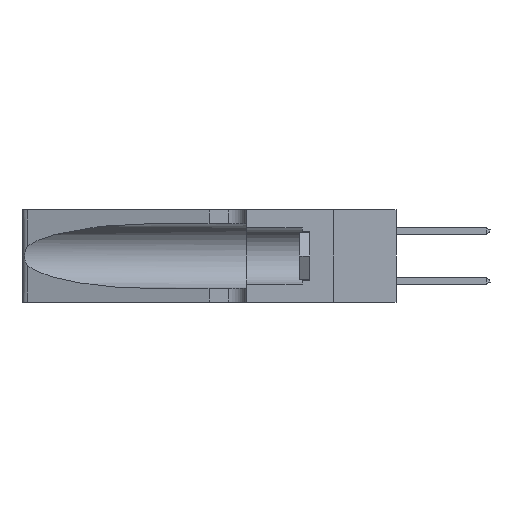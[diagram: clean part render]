
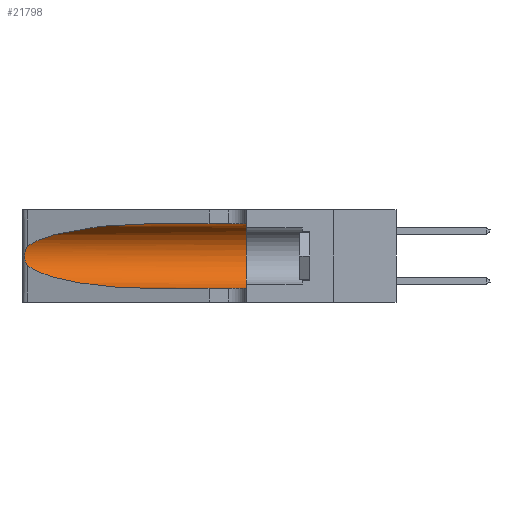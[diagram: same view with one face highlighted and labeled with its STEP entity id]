
A CAD part, left-side view. The second image highlights one B-rep face of the part: STEP entity #21798.
In plain terms, the highlighted cylindrical face has radius 3.308 mm (diameter 6.617 mm), a partial arc.
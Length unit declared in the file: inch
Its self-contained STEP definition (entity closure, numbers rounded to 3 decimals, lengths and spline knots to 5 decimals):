
#53 = CARTESIAN_POINT ( 'NONE',  ( 0.1305, 1.61858, 0.05475 ) ) ;
#1114 = CARTESIAN_POINT ( 'NONE',  ( 0.26075, 1.23896, 0.19203 ) ) ;
#1781 =( BOUNDED_CURVE ( )  B_SPLINE_CURVE ( 3, ( #29916, #9911, #32738, #15799 ),
 .UNSPECIFIED., .F., .F. ) 
 B_SPLINE_CURVE_WITH_KNOTS ( ( 4, 4 ),
 ( 1.5708, 2.84003 ),
 .UNSPECIFIED. ) 
 CURVE ( )  GEOMETRIC_REPRESENTATION_ITEM ( )  RATIONAL_B_SPLINE_CURVE ( ( 1., 0.87, 0.87, 1. ) ) 
 REPRESENTATION_ITEM ( '' )  );
#2050 = AXIS2_PLACEMENT_3D ( 'NONE', #6379, #26395, #9287 ) ;
#2998 = EDGE_LOOP ( 'NONE', ( #20189, #3966, #34275, #18546, #19364, #13245 ) ) ;
#3966 = ORIENTED_EDGE ( 'NONE', *, *, #14239, .T. ) ;
#4120 = CARTESIAN_POINT ( 'NONE',  ( 0.26017, 1.23833, 0.17102 ) ) ;
#4672 = B_SPLINE_CURVE_WITH_KNOTS ( 'NONE', 3,
 ( #24072, #9840, #32544, #15597, #35403, #18487, #1114, #21344, #4120, #24201, #7073, #27046, #9971, #29843 ),
 .UNSPECIFIED., .F., .F.,
 ( 4, 2, 2, 2, 2, 2, 4 ),
 ( 0., 0.00027, 0.00053, 0.00107, 0.0016, 0.00187, 0.00214 ),
 .UNSPECIFIED. ) ;
#4961 = VERTEX_POINT ( 'NONE', #33098 ) ;
#5227 = VERTEX_POINT ( 'NONE', #11500 ) ;
#5670 = CARTESIAN_POINT ( 'NONE',  ( 0.1305, 1.61858, 0.31525 ) ) ;
#6115 = CARTESIAN_POINT ( 'NONE',  ( 0.1305, 0.72297, 0.05475 ) ) ;
#6379 = CARTESIAN_POINT ( 'NONE',  ( 0.1305, 0.35, 0.185 ) ) ;
#7073 = CARTESIAN_POINT ( 'NONE',  ( 0.25789, 1.23486, 0.15765 ) ) ;
#9287 = DIRECTION ( 'NONE',  ( 0., 0., 1. ) ) ;
#9401 = CARTESIAN_POINT ( 'NONE',  ( 0.1305, 1.61858, 0.185 ) ) ;
#9840 = CARTESIAN_POINT ( 'NONE',  ( 0.25555, 1.22994, 0.2215 ) ) ;
#9911 = CARTESIAN_POINT ( 'NONE',  ( 0.18966, 0.96281, 0.31525 ) ) ;
#9971 = CARTESIAN_POINT ( 'NONE',  ( 0.25555, 1.22993, 0.14849 ) ) ;
#10057 = EDGE_CURVE ( 'NONE', #14103, #4961, #18023, .T. ) ;
#11257 = CARTESIAN_POINT ( 'NONE',  ( 0.1305, 0.35, 0.31525 ) ) ;
#11417 = CARTESIAN_POINT ( 'NONE',  ( 0.25487, 1.22718, 0.22369 ) ) ;
#11500 = CARTESIAN_POINT ( 'NONE',  ( 0.1305, 0.72297, 0.31525 ) ) ;
#11599 = CARTESIAN_POINT ( 'NONE',  ( 0.25487, 1.22718, 0.14631 ) ) ;
#12283 = DIRECTION ( 'NONE',  ( 0., -1., 0. ) ) ;
#13133 = CYLINDRICAL_SURFACE ( 'NONE', #27739, 0.13025 ) ;
#13245 = ORIENTED_EDGE ( 'NONE', *, *, #31422, .F. ) ;
#14103 = VERTEX_POINT ( 'NONE', #11599 ) ;
#14217 = DIRECTION ( 'NONE',  ( 0., -1., 0. ) ) ;
#14239 = EDGE_CURVE ( 'NONE', #15331, #14103, #4672, .T. ) ;
#14615 = DIRECTION ( 'NONE',  ( 0., -1., 0. ) ) ;
#14776 = VERTEX_POINT ( 'NONE', #23659 ) ;
#15331 = VERTEX_POINT ( 'NONE', #11417 ) ;
#15597 = CARTESIAN_POINT ( 'NONE',  ( 0.25787, 1.23484, 0.2124 ) ) ;
#15799 = CARTESIAN_POINT ( 'NONE',  ( 0.25487, 1.22718, 0.22369 ) ) ;
#18023 =( BOUNDED_CURVE ( )  B_SPLINE_CURVE ( 3, ( #26009, #23145, #23266, #6115 ),
 .UNSPECIFIED., .F., .T. ) 
 B_SPLINE_CURVE_WITH_KNOTS ( ( 4, 4 ),
 ( 3.44316, 4.71239 ),
 .UNSPECIFIED. ) 
 CURVE ( )  GEOMETRIC_REPRESENTATION_ITEM ( )  RATIONAL_B_SPLINE_CURVE ( ( 1., 0.87, 0.87, 1. ) ) 
 REPRESENTATION_ITEM ( '' )  );
#18487 = CARTESIAN_POINT ( 'NONE',  ( 0.26018, 1.23835, 0.19895 ) ) ;
#18546 = ORIENTED_EDGE ( 'NONE', *, *, #20034, .T. ) ;
#19364 = ORIENTED_EDGE ( 'NONE', *, *, #35878, .F. ) ;
#19437 = CIRCLE ( 'NONE', #2050, 0.13025 ) ;
#20034 = EDGE_CURVE ( 'NONE', #4961, #14776, #27897, .T. ) ;
#20189 = ORIENTED_EDGE ( 'NONE', *, *, #25973, .T. ) ;
#21055 = LINE ( 'NONE', #5670, #27699 ) ;
#21344 = CARTESIAN_POINT ( 'NONE',  ( 0.26075, 1.23896, 0.178 ) ) ;
#21798 = ADVANCED_FACE ( 'NONE', ( #35739 ), #13133, .F. ) ;
#22828 = VERTEX_POINT ( 'NONE', #11257 ) ;
#23145 = CARTESIAN_POINT ( 'NONE',  ( 0.2373, 1.15595, 0.08982 ) ) ;
#23266 = CARTESIAN_POINT ( 'NONE',  ( 0.18966, 0.96281, 0.05475 ) ) ;
#23659 = CARTESIAN_POINT ( 'NONE',  ( 0.1305, 0.35, 0.05475 ) ) ;
#24072 = CARTESIAN_POINT ( 'NONE',  ( 0.25487, 1.22718, 0.22369 ) ) ;
#24201 = CARTESIAN_POINT ( 'NONE',  ( 0.25856, 1.23593, 0.16098 ) ) ;
#25973 = EDGE_CURVE ( 'NONE', #5227, #15331, #1781, .T. ) ;
#26009 = CARTESIAN_POINT ( 'NONE',  ( 0.25487, 1.22718, 0.14631 ) ) ;
#26395 = DIRECTION ( 'NONE',  ( 0., 1., 0. ) ) ;
#26503 = DIRECTION ( 'NONE',  ( 0., 0., -1. ) ) ;
#27046 = CARTESIAN_POINT ( 'NONE',  ( 0.25639, 1.23186, 0.15144 ) ) ;
#27699 = VECTOR ( 'NONE', #14217, 39.37008 ) ;
#27739 = AXIS2_PLACEMENT_3D ( 'NONE', #9401, #12283, #26503 ) ;
#27897 = LINE ( 'NONE', #53, #36269 ) ;
#29843 = CARTESIAN_POINT ( 'NONE',  ( 0.25487, 1.22718, 0.14631 ) ) ;
#29916 = CARTESIAN_POINT ( 'NONE',  ( 0.1305, 0.72297, 0.31525 ) ) ;
#31422 = EDGE_CURVE ( 'NONE', #5227, #22828, #21055, .T. ) ;
#32544 = CARTESIAN_POINT ( 'NONE',  ( 0.25639, 1.23184, 0.21858 ) ) ;
#32738 = CARTESIAN_POINT ( 'NONE',  ( 0.2373, 1.15595, 0.28018 ) ) ;
#33098 = CARTESIAN_POINT ( 'NONE',  ( 0.1305, 0.72297, 0.05475 ) ) ;
#34275 = ORIENTED_EDGE ( 'NONE', *, *, #10057, .T. ) ;
#35403 = CARTESIAN_POINT ( 'NONE',  ( 0.25854, 1.2359, 0.20912 ) ) ;
#35739 = FACE_OUTER_BOUND ( 'NONE', #2998, .T. ) ;
#35878 = EDGE_CURVE ( 'NONE', #22828, #14776, #19437, .T. ) ;
#36269 = VECTOR ( 'NONE', #14615, 39.37008 ) ;
